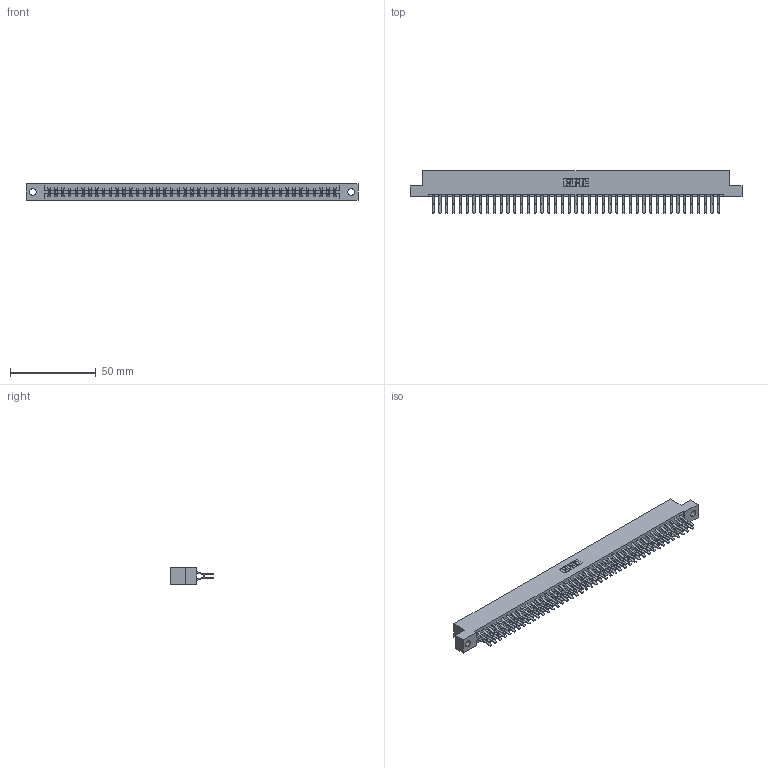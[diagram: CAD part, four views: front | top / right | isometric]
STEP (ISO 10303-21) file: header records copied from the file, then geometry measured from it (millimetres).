
FILE_DESCRIPTION (( 'STEP AP203' ), '1' );
FILE_NAME ('337-086-560-204.STEP', '2018-08-13T02:38:44', ( '' ), ( '' ), 'SwSTEP 2.0', 'SolidWorks 2016', '' );
FILE_SCHEMA (( 'CONFIG_CONTROL_DESIGN' ));
Length unit declared in the file: inch
Products named in the file (3): 337 Part_Flush Mounting Lugs - 0.156 Dia-TH; 345-292-001_560 Tail; 337-086-560-204
Assembly tree (87 placements, depth 2):
  337-086-560-204
    337 Part_Flush Mounting Lugs - 0.156 Dia-TH
    345-292-001_560 Tail  x86
Bounding box: 193.4 x 24.78 x 9.4 mm (x, y, z)
Volume: 20870.7 mm3; surface area: 25033 mm2
Topology: 87 solids, 87 shells, 4930 faces, 14673 edges, 9666 vertices
Faces by surface type: plane 3338, cylinder 1592
Entity records: 33301 total; most frequent: CARTESIAN_POINT 5610, ORIENTED_EDGE 5546, DIRECTION 4773, EDGE_CURVE 2773, LINE 2641, VECTOR 2641, VERTEX_POINT 1846, AXIS2_PLACEMENT_3D 1066
